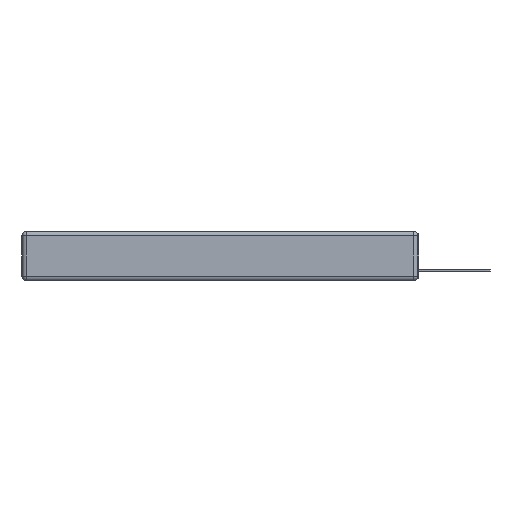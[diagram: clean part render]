
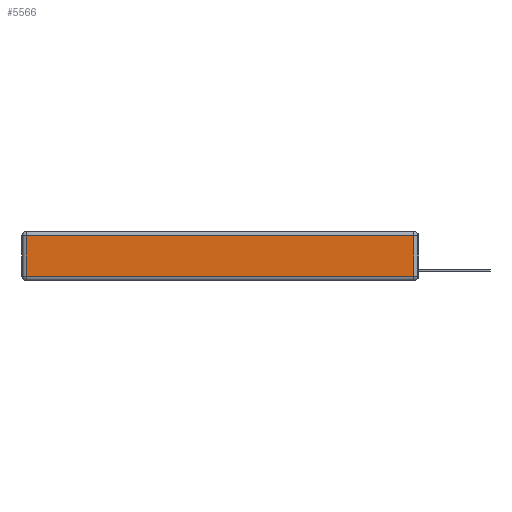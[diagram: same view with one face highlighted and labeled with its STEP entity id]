
A CAD part, left-side view. The second image highlights one B-rep face of the part: STEP entity #5566.
In plain terms, the highlighted planar face has unit normal (-1, 0, 0).
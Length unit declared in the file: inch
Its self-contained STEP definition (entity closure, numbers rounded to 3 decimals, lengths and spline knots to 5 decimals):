
#228 = DIRECTION ( 'NONE',  ( 0., 1., 0. ) ) ;
#1156 = PLANE ( 'NONE',  #3900 ) ;
#1517 = CARTESIAN_POINT ( 'NONE',  ( 0., 0., -0.313 ) ) ;
#1666 = VERTEX_POINT ( 'NONE', #22544 ) ;
#1974 = DIRECTION ( 'NONE',  ( 0., 0., 1. ) ) ;
#3619 = LINE ( 'NONE', #10727, #13220 ) ;
#3900 = AXIS2_PLACEMENT_3D ( 'NONE', #13423, #4699, #16920 ) ;
#4085 = VERTEX_POINT ( 'NONE', #4087 ) ;
#4087 = CARTESIAN_POINT ( 'NONE',  ( 0., 0.03, -0.313 ) ) ;
#4699 = DIRECTION ( 'NONE',  ( -1., 0., 0. ) ) ;
#4700 = EDGE_CURVE ( 'NONE', #8188, #1666, #3619, .T. ) ;
#4708 = FACE_OUTER_BOUND ( 'NONE', #13252, .T. ) ;
#5566 = ADVANCED_FACE ( 'NONE', ( #4708 ), #1156, .T. ) ;
#6185 = CARTESIAN_POINT ( 'NONE',  ( 0., 0.03, -0.03 ) ) ;
#8015 = VECTOR ( 'NONE', #1974, 39.37008 ) ;
#8188 = VERTEX_POINT ( 'NONE', #6185 ) ;
#8892 = CARTESIAN_POINT ( 'NONE',  ( 0., 0.03, -0.343 ) ) ;
#9749 = ORIENTED_EDGE ( 'NONE', *, *, #14064, .T. ) ;
#10727 = CARTESIAN_POINT ( 'NONE',  ( 0., 2.75, -0.03 ) ) ;
#12868 = ORIENTED_EDGE ( 'NONE', *, *, #4700, .T. ) ;
#13094 = LINE ( 'NONE', #1517, #13386 ) ;
#13220 = VECTOR ( 'NONE', #228, 39.37008 ) ;
#13252 = EDGE_LOOP ( 'NONE', ( #15297, #9749, #12868, #19012 ) ) ;
#13386 = VECTOR ( 'NONE', #22348, 39.37008 ) ;
#13423 = CARTESIAN_POINT ( 'NONE',  ( 0., 0., -0.343 ) ) ;
#13827 = CARTESIAN_POINT ( 'NONE',  ( 0., 2.72, -0.313 ) ) ;
#14064 = EDGE_CURVE ( 'NONE', #4085, #8188, #15635, .T. ) ;
#14392 = LINE ( 'NONE', #18120, #18502 ) ;
#15297 = ORIENTED_EDGE ( 'NONE', *, *, #15797, .T. ) ;
#15635 = LINE ( 'NONE', #8892, #8015 ) ;
#15797 = EDGE_CURVE ( 'NONE', #17860, #4085, #13094, .T. ) ;
#16587 = DIRECTION ( 'NONE',  ( 0., 0., -1. ) ) ;
#16920 = DIRECTION ( 'NONE',  ( 0., 0., 1. ) ) ;
#17860 = VERTEX_POINT ( 'NONE', #13827 ) ;
#18120 = CARTESIAN_POINT ( 'NONE',  ( 0., 2.72, -0.343 ) ) ;
#18502 = VECTOR ( 'NONE', #16587, 39.37008 ) ;
#19012 = ORIENTED_EDGE ( 'NONE', *, *, #22212, .T. ) ;
#22212 = EDGE_CURVE ( 'NONE', #1666, #17860, #14392, .T. ) ;
#22348 = DIRECTION ( 'NONE',  ( 0., -1., 0. ) ) ;
#22544 = CARTESIAN_POINT ( 'NONE',  ( 0., 2.72, -0.03 ) ) ;
